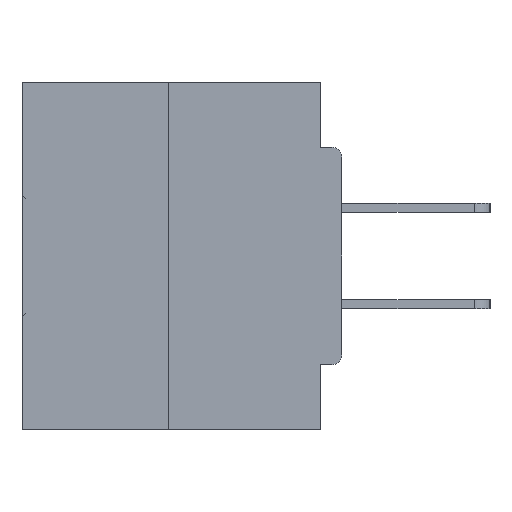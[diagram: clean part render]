
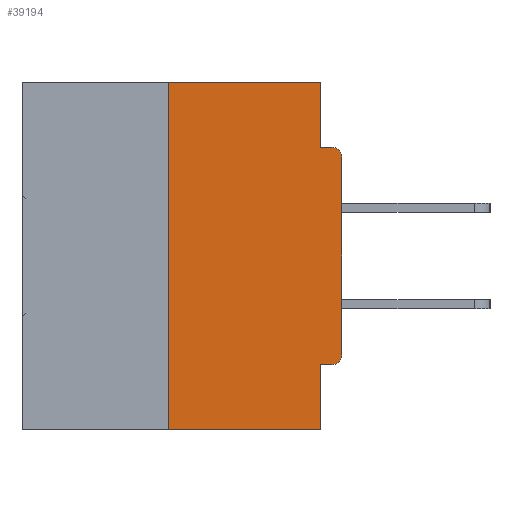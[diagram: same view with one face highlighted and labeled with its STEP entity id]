
A CAD part, left-side view. The second image highlights one B-rep face of the part: STEP entity #39194.
In plain terms, the highlighted planar face has unit normal (-1, 0, 0).
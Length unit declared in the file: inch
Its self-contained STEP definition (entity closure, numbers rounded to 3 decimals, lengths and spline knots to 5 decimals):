
#159 = EDGE_CURVE ( 'NONE', #1927, #15016, #15059, .T. ) ;
#461 = AXIS2_PLACEMENT_3D ( 'NONE', #38301, #34752, #25170 ) ;
#583 = FACE_OUTER_BOUND ( 'NONE', #22183, .T. ) ;
#1927 = VERTEX_POINT ( 'NONE', #19667 ) ;
#2066 = AXIS2_PLACEMENT_3D ( 'NONE', #41938, #21510, #11553 ) ;
#2438 = CARTESIAN_POINT ( 'NONE',  ( 0., 0.25, 0. ) ) ;
#3400 = VERTEX_POINT ( 'NONE', #10819 ) ;
#3583 = VERTEX_POINT ( 'NONE', #12337 ) ;
#5275 = LINE ( 'NONE', #39223, #20824 ) ;
#6037 = DIRECTION ( 'NONE',  ( 0., 1., 0. ) ) ;
#6209 = EDGE_CURVE ( 'NONE', #7483, #10419, #15303, .T. ) ;
#6305 = ORIENTED_EDGE ( 'NONE', *, *, #43773, .T. ) ;
#6903 = DIRECTION ( 'NONE',  ( 0., 0., -1. ) ) ;
#6968 = CARTESIAN_POINT ( 'NONE',  ( 0., 0., -0.0935 ) ) ;
#7483 = VERTEX_POINT ( 'NONE', #2438 ) ;
#8239 = ORIENTED_EDGE ( 'NONE', *, *, #42235, .T. ) ;
#8615 = DIRECTION ( 'NONE',  ( 0., 0., -1. ) ) ;
#9098 = CARTESIAN_POINT ( 'NONE',  ( 0., 0.46, 0. ) ) ;
#9106 = VERTEX_POINT ( 'NONE', #33488 ) ;
#10419 = VERTEX_POINT ( 'NONE', #25524 ) ;
#10530 = ORIENTED_EDGE ( 'NONE', *, *, #12428, .F. ) ;
#10819 = CARTESIAN_POINT ( 'NONE',  ( 0., 0., -0.3915 ) ) ;
#11553 = DIRECTION ( 'NONE',  ( 0., 0., -1. ) ) ;
#11671 = PLANE ( 'NONE',  #461 ) ;
#11976 = DIRECTION ( 'NONE',  ( 0., -1., 0. ) ) ;
#12337 = CARTESIAN_POINT ( 'NONE',  ( 0., 0.015, -0.0935 ) ) ;
#12428 = EDGE_CURVE ( 'NONE', #23972, #3583, #27576, .T. ) ;
#13957 = ORIENTED_EDGE ( 'NONE', *, *, #23127, .F. ) ;
#14045 = AXIS2_PLACEMENT_3D ( 'NONE', #29758, #43313, #6903 ) ;
#14289 = ORIENTED_EDGE ( 'NONE', *, *, #43357, .F. ) ;
#15016 = VERTEX_POINT ( 'NONE', #15712 ) ;
#15059 = LINE ( 'NONE', #41682, #36616 ) ;
#15303 = LINE ( 'NONE', #9098, #38476 ) ;
#15712 = CARTESIAN_POINT ( 'NONE',  ( 0., 0.031, -0.5 ) ) ;
#16742 = CARTESIAN_POINT ( 'NONE',  ( 0., 0.031, -0.0935 ) ) ;
#17249 = LINE ( 'NONE', #30787, #25205 ) ;
#17376 = DIRECTION ( 'NONE',  ( 0., -1., 0. ) ) ;
#18622 = DIRECTION ( 'NONE',  ( 0., 0., 1. ) ) ;
#18700 = EDGE_CURVE ( 'NONE', #42836, #15016, #22460, .T. ) ;
#19497 = CARTESIAN_POINT ( 'NONE',  ( 0., 0.25, 0. ) ) ;
#19667 = CARTESIAN_POINT ( 'NONE',  ( 0., 0.031, -0.4065 ) ) ;
#19760 = VECTOR ( 'NONE', #6037, 39.37008 ) ;
#20824 = VECTOR ( 'NONE', #8615, 39.37008 ) ;
#21143 = ORIENTED_EDGE ( 'NONE', *, *, #34118, .T. ) ;
#21510 = DIRECTION ( 'NONE',  ( -1., 0., 0. ) ) ;
#22183 = EDGE_LOOP ( 'NONE', ( #40526, #32692, #35861, #29022, #14289, #6305, #21143, #8239, #10530, #13957 ) ) ;
#22460 = LINE ( 'NONE', #29350, #39637 ) ;
#22620 = VECTOR ( 'NONE', #18622, 39.37008 ) ;
#23127 = EDGE_CURVE ( 'NONE', #10419, #23972, #5275, .T. ) ;
#23359 = VERTEX_POINT ( 'NONE', #24482 ) ;
#23972 = VERTEX_POINT ( 'NONE', #16742 ) ;
#24482 = CARTESIAN_POINT ( 'NONE',  ( 0., 0., -0.1085 ) ) ;
#25170 = DIRECTION ( 'NONE',  ( 0., 0., -1. ) ) ;
#25205 = VECTOR ( 'NONE', #30995, 39.37008 ) ;
#25446 = DIRECTION ( 'NONE',  ( 0., 0., -1. ) ) ;
#25524 = CARTESIAN_POINT ( 'NONE',  ( 0., 0.031, 0. ) ) ;
#25540 = CARTESIAN_POINT ( 'NONE',  ( 0., 0., -0.4065 ) ) ;
#25582 = VECTOR ( 'NONE', #17376, 39.37008 ) ;
#27453 = CARTESIAN_POINT ( 'NONE',  ( 0., 0.25, -0.5 ) ) ;
#27576 = LINE ( 'NONE', #6968, #25582 ) ;
#29022 = ORIENTED_EDGE ( 'NONE', *, *, #159, .F. ) ;
#29350 = CARTESIAN_POINT ( 'NONE',  ( 0., 0.46, -0.5 ) ) ;
#29758 = CARTESIAN_POINT ( 'NONE',  ( 0., 0.015, -0.1085 ) ) ;
#30787 = CARTESIAN_POINT ( 'NONE',  ( 0., 0., 0. ) ) ;
#30995 = DIRECTION ( 'NONE',  ( 0., 0., 1. ) ) ;
#31852 = CIRCLE ( 'NONE', #2066, 0.015 ) ;
#32692 = ORIENTED_EDGE ( 'NONE', *, *, #33440, .F. ) ;
#33440 = EDGE_CURVE ( 'NONE', #42836, #7483, #39704, .T. ) ;
#33488 = CARTESIAN_POINT ( 'NONE',  ( 0., 0.015, -0.4065 ) ) ;
#34118 = EDGE_CURVE ( 'NONE', #3400, #23359, #17249, .T. ) ;
#34752 = DIRECTION ( 'NONE',  ( 1., 0., 0. ) ) ;
#35298 = CIRCLE ( 'NONE', #14045, 0.015 ) ;
#35861 = ORIENTED_EDGE ( 'NONE', *, *, #18700, .T. ) ;
#36020 = DIRECTION ( 'NONE',  ( 0., -1., 0. ) ) ;
#36616 = VECTOR ( 'NONE', #25446, 39.37008 ) ;
#38301 = CARTESIAN_POINT ( 'NONE',  ( 0., 0.46, 0. ) ) ;
#38476 = VECTOR ( 'NONE', #11976, 39.37008 ) ;
#39194 = ADVANCED_FACE ( 'NONE', ( #583 ), #11671, .F. ) ;
#39223 = CARTESIAN_POINT ( 'NONE',  ( 0., 0.031, 0. ) ) ;
#39637 = VECTOR ( 'NONE', #36020, 39.37008 ) ;
#39704 = LINE ( 'NONE', #19497, #22620 ) ;
#40526 = ORIENTED_EDGE ( 'NONE', *, *, #6209, .F. ) ;
#41682 = CARTESIAN_POINT ( 'NONE',  ( 0., 0.031, -0.5 ) ) ;
#41938 = CARTESIAN_POINT ( 'NONE',  ( 0., 0.015, -0.3915 ) ) ;
#42235 = EDGE_CURVE ( 'NONE', #23359, #3583, #35298, .T. ) ;
#42836 = VERTEX_POINT ( 'NONE', #27453 ) ;
#43313 = DIRECTION ( 'NONE',  ( -1., 0., 0. ) ) ;
#43321 = LINE ( 'NONE', #25540, #19760 ) ;
#43357 = EDGE_CURVE ( 'NONE', #9106, #1927, #43321, .T. ) ;
#43773 = EDGE_CURVE ( 'NONE', #9106, #3400, #31852, .T. ) ;
